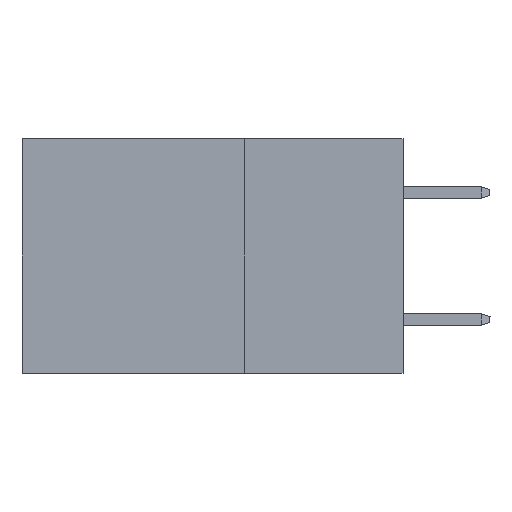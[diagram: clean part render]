
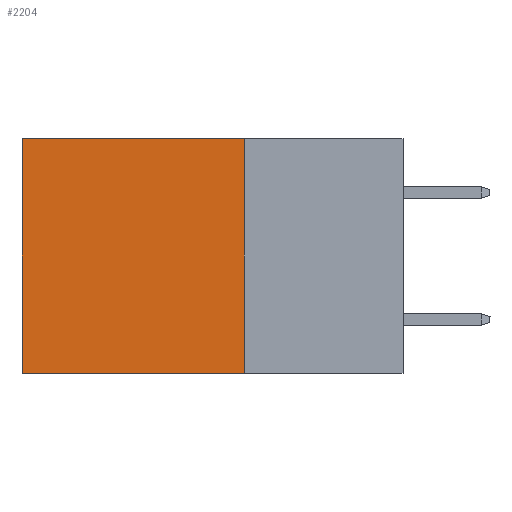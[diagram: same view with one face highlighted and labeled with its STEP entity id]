
A CAD part, left-side view. The second image highlights one B-rep face of the part: STEP entity #2204.
In plain terms, the highlighted planar face has unit normal (-1, 0, 0).
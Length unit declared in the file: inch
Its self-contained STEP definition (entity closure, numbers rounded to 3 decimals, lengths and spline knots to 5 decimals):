
#359 = DIRECTION ( 'NONE',  ( 0., 1., 0. ) ) ;
#1980 = EDGE_CURVE ( 'NONE', #12178, #5105, #30316, .T. ) ;
#2204 = ADVANCED_FACE ( 'NONE', ( #5477 ), #21411, .F. ) ;
#2847 = LINE ( 'NONE', #23304, #32835 ) ;
#3061 = LINE ( 'NONE', #23340, #25550 ) ;
#3134 = VERTEX_POINT ( 'NONE', #19397 ) ;
#3562 = ORIENTED_EDGE ( 'NONE', *, *, #1980, .T. ) ;
#4020 = AXIS2_PLACEMENT_3D ( 'NONE', #31584, #15547, #31238 ) ;
#5105 = VERTEX_POINT ( 'NONE', #15629 ) ;
#5404 = DIRECTION ( 'NONE',  ( 0., 0., -1. ) ) ;
#5477 = FACE_OUTER_BOUND ( 'NONE', #9610, .T. ) ;
#6158 = VECTOR ( 'NONE', #17623, 39.37008 ) ;
#7095 = EDGE_CURVE ( 'NONE', #5105, #15207, #3061, .T. ) ;
#7401 = CARTESIAN_POINT ( 'NONE',  ( 0.2875, 0.25, 0. ) ) ;
#9610 = EDGE_LOOP ( 'NONE', ( #27177, #15469, #24650, #3562 ) ) ;
#12178 = VERTEX_POINT ( 'NONE', #22372 ) ;
#12727 = EDGE_CURVE ( 'NONE', #12178, #3134, #18732, .T. ) ;
#15207 = VERTEX_POINT ( 'NONE', #15595 ) ;
#15469 = ORIENTED_EDGE ( 'NONE', *, *, #23718, .F. ) ;
#15547 = DIRECTION ( 'NONE',  ( 1., 0., 0. ) ) ;
#15595 = CARTESIAN_POINT ( 'NONE',  ( 0.2875, 0.6, -0.37 ) ) ;
#15629 = CARTESIAN_POINT ( 'NONE',  ( 0.2875, 0.6, 0. ) ) ;
#17623 = DIRECTION ( 'NONE',  ( 0., 1., 0. ) ) ;
#18732 = LINE ( 'NONE', #28924, #28926 ) ;
#19397 = CARTESIAN_POINT ( 'NONE',  ( 0.2875, 0.25, -0.37 ) ) ;
#21411 = PLANE ( 'NONE',  #4020 ) ;
#22372 = CARTESIAN_POINT ( 'NONE',  ( 0.2875, 0.25, 0. ) ) ;
#23304 = CARTESIAN_POINT ( 'NONE',  ( 0.2875, 0.25, -0.37 ) ) ;
#23340 = CARTESIAN_POINT ( 'NONE',  ( 0.2875, 0.6, 0. ) ) ;
#23718 = EDGE_CURVE ( 'NONE', #3134, #15207, #2847, .T. ) ;
#24650 = ORIENTED_EDGE ( 'NONE', *, *, #12727, .F. ) ;
#25550 = VECTOR ( 'NONE', #5404, 39.37008 ) ;
#26416 = DIRECTION ( 'NONE',  ( 0., 0., -1. ) ) ;
#27177 = ORIENTED_EDGE ( 'NONE', *, *, #7095, .T. ) ;
#28924 = CARTESIAN_POINT ( 'NONE',  ( 0.2875, 0.25, 0. ) ) ;
#28926 = VECTOR ( 'NONE', #26416, 39.37008 ) ;
#30316 = LINE ( 'NONE', #7401, #6158 ) ;
#31238 = DIRECTION ( 'NONE',  ( 0., 0., -1. ) ) ;
#31584 = CARTESIAN_POINT ( 'NONE',  ( 0.2875, 0.25, 0. ) ) ;
#32835 = VECTOR ( 'NONE', #359, 39.37008 ) ;
